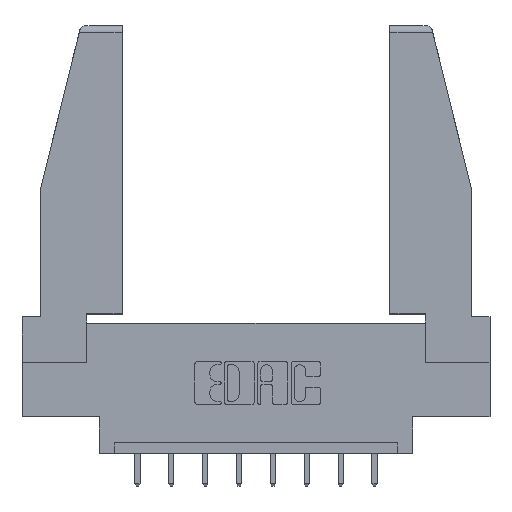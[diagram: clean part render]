
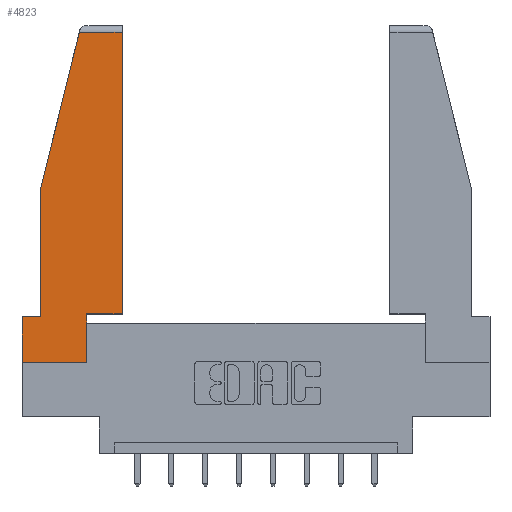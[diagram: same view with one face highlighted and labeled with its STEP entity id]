
A CAD part, top view. The second image highlights one B-rep face of the part: STEP entity #4823.
In plain terms, the highlighted planar face has unit normal (0, 0, 1).
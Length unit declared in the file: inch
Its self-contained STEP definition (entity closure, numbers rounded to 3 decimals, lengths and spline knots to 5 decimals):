
#233 = CARTESIAN_POINT ( 'NONE',  ( 0., 1.52, 0. ) ) ;
#257 = LINE ( 'NONE', #12618, #9135 ) ;
#467 = ORIENTED_EDGE ( 'NONE', *, *, #11144, .T. ) ;
#505 = CARTESIAN_POINT ( 'NONE',  ( 0.086, 0.8, 0. ) ) ;
#548 = CARTESIAN_POINT ( 'NONE',  ( 0.461, 0.223, 0. ) ) ;
#808 = EDGE_CURVE ( 'NONE', #4876, #8568, #6503, .T. ) ;
#860 = CARTESIAN_POINT ( 'NONE',  ( 0., 0.21, 0. ) ) ;
#933 = CARTESIAN_POINT ( 'NONE',  ( 0.297, 0.223, 0. ) ) ;
#1046 = EDGE_CURVE ( 'NONE', #2978, #9726, #2784, .T. ) ;
#1175 = VECTOR ( 'NONE', #4257, 39.37008 ) ;
#1438 = VECTOR ( 'NONE', #1981, 39.37008 ) ;
#1981 = DIRECTION ( 'NONE',  ( -1., 0., 0. ) ) ;
#2332 = DIRECTION ( 'NONE',  ( 1., 0., 0. ) ) ;
#2784 = LINE ( 'NONE', #233, #12478 ) ;
#2978 = VERTEX_POINT ( 'NONE', #7725 ) ;
#3019 = VECTOR ( 'NONE', #8543, 39.37008 ) ;
#3084 = ORIENTED_EDGE ( 'NONE', *, *, #6912, .T. ) ;
#3192 = CARTESIAN_POINT ( 'NONE',  ( 0.297, 0., 0. ) ) ;
#3255 = ORIENTED_EDGE ( 'NONE', *, *, #808, .T. ) ;
#3293 = VERTEX_POINT ( 'NONE', #7679 ) ;
#3323 = ORIENTED_EDGE ( 'NONE', *, *, #4268, .T. ) ;
#3434 = EDGE_CURVE ( 'NONE', #8548, #4016, #257, .T. ) ;
#3445 = CARTESIAN_POINT ( 'NONE',  ( 0.086, 0.8, 0. ) ) ;
#4016 = VERTEX_POINT ( 'NONE', #6872 ) ;
#4107 = LINE ( 'NONE', #860, #1438 ) ;
#4257 = DIRECTION ( 'NONE',  ( 1., 0., 0. ) ) ;
#4268 = EDGE_CURVE ( 'NONE', #8568, #11002, #8809, .T. ) ;
#4340 = VERTEX_POINT ( 'NONE', #3445 ) ;
#4562 = DIRECTION ( 'NONE',  ( 0., 1., 0. ) ) ;
#4823 = ADVANCED_FACE ( 'NONE', ( #8294 ), #11218, .T. ) ;
#4876 = VERTEX_POINT ( 'NONE', #6294 ) ;
#4926 = VECTOR ( 'NONE', #12371, 39.37008 ) ;
#5352 = EDGE_CURVE ( 'NONE', #9726, #4340, #10190, .T. ) ;
#5520 = EDGE_CURVE ( 'NONE', #3293, #4876, #4107, .T. ) ;
#5608 = ORIENTED_EDGE ( 'NONE', *, *, #3434, .T. ) ;
#5936 = LINE ( 'NONE', #505, #8242 ) ;
#6030 = AXIS2_PLACEMENT_3D ( 'NONE', #7309, #10162, #2332 ) ;
#6097 = DIRECTION ( 'NONE',  ( -1., 0., 0. ) ) ;
#6294 = CARTESIAN_POINT ( 'NONE',  ( 0., 0.21, 0. ) ) ;
#6409 = LINE ( 'NONE', #9748, #3019 ) ;
#6503 = LINE ( 'NONE', #6640, #11091 ) ;
#6640 = CARTESIAN_POINT ( 'NONE',  ( 0., 0.21, 0. ) ) ;
#6826 = ORIENTED_EDGE ( 'NONE', *, *, #5352, .T. ) ;
#6872 = CARTESIAN_POINT ( 'NONE',  ( 0.461, 0.223, 0. ) ) ;
#6912 = EDGE_CURVE ( 'NONE', #4016, #2978, #9463, .T. ) ;
#7309 = CARTESIAN_POINT ( 'NONE',  ( 0., 0., 0. ) ) ;
#7679 = CARTESIAN_POINT ( 'NONE',  ( 0.086, 0.21, 0. ) ) ;
#7725 = CARTESIAN_POINT ( 'NONE',  ( 0.461, 1.52, 0. ) ) ;
#7736 = EDGE_LOOP ( 'NONE', ( #3084, #11186, #6826, #467, #10323, #3255, #3323, #8711, #5608 ) ) ;
#8242 = VECTOR ( 'NONE', #12584, 39.37008 ) ;
#8294 = FACE_OUTER_BOUND ( 'NONE', #7736, .T. ) ;
#8543 = DIRECTION ( 'NONE',  ( 0., 1., 0. ) ) ;
#8548 = VERTEX_POINT ( 'NONE', #933 ) ;
#8568 = VERTEX_POINT ( 'NONE', #11312 ) ;
#8711 = ORIENTED_EDGE ( 'NONE', *, *, #8953, .T. ) ;
#8809 = LINE ( 'NONE', #9293, #1175 ) ;
#8953 = EDGE_CURVE ( 'NONE', #11002, #8548, #6409, .T. ) ;
#9135 = VECTOR ( 'NONE', #11714, 39.37008 ) ;
#9293 = CARTESIAN_POINT ( 'NONE',  ( 0., 0., 0. ) ) ;
#9463 = LINE ( 'NONE', #548, #9796 ) ;
#9726 = VERTEX_POINT ( 'NONE', #11375 ) ;
#9731 = DIRECTION ( 'NONE',  ( 0., -1., 0. ) ) ;
#9748 = CARTESIAN_POINT ( 'NONE',  ( 0.297, 0., 0. ) ) ;
#9796 = VECTOR ( 'NONE', #4562, 39.37008 ) ;
#10162 = DIRECTION ( 'NONE',  ( 0., 0., 1. ) ) ;
#10190 = LINE ( 'NONE', #10443, #4926 ) ;
#10323 = ORIENTED_EDGE ( 'NONE', *, *, #5520, .T. ) ;
#10443 = CARTESIAN_POINT ( 'NONE',  ( 0.271, 1.55, 0. ) ) ;
#11002 = VERTEX_POINT ( 'NONE', #3192 ) ;
#11091 = VECTOR ( 'NONE', #9731, 39.37008 ) ;
#11144 = EDGE_CURVE ( 'NONE', #4340, #3293, #5936, .T. ) ;
#11186 = ORIENTED_EDGE ( 'NONE', *, *, #1046, .T. ) ;
#11218 = PLANE ( 'NONE',  #6030 ) ;
#11312 = CARTESIAN_POINT ( 'NONE',  ( 0., 0., 0. ) ) ;
#11375 = CARTESIAN_POINT ( 'NONE',  ( 0.2636, 1.52, 0. ) ) ;
#11714 = DIRECTION ( 'NONE',  ( 1., 0., 0. ) ) ;
#12371 = DIRECTION ( 'NONE',  ( -0.239, -0.971, 0. ) ) ;
#12478 = VECTOR ( 'NONE', #6097, 39.37008 ) ;
#12584 = DIRECTION ( 'NONE',  ( 0., -1., 0. ) ) ;
#12618 = CARTESIAN_POINT ( 'NONE',  ( 0.297, 0.223, 0. ) ) ;
